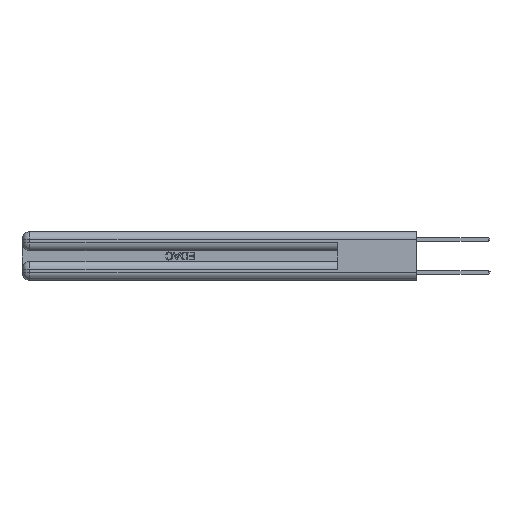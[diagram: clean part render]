
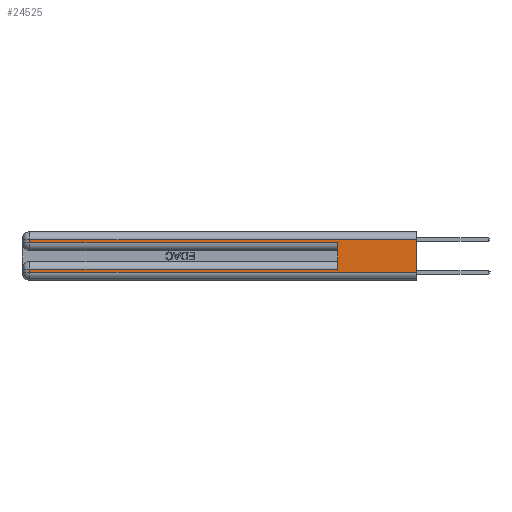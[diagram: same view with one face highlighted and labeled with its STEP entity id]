
A CAD part, left-side view. The second image highlights one B-rep face of the part: STEP entity #24525.
In plain terms, the highlighted planar face has unit normal (-1, 0, 0).
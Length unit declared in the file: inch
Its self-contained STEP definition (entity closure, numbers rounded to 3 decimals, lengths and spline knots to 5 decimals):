
#641 = CARTESIAN_POINT ( 'NONE',  ( 0., 0., 0.37 ) ) ;
#754 = DIRECTION ( 'NONE',  ( 0., 0., 1. ) ) ;
#1929 = CARTESIAN_POINT ( 'NONE',  ( 0., 2.94, 0.285 ) ) ;
#3793 = LINE ( 'NONE', #35618, #17306 ) ;
#3908 = DIRECTION ( 'NONE',  ( 0., 0., -1. ) ) ;
#4179 = EDGE_CURVE ( 'NONE', #4597, #15960, #12061, .T. ) ;
#4214 = CARTESIAN_POINT ( 'NONE',  ( 0., 0.6, 0.285 ) ) ;
#4295 = ORIENTED_EDGE ( 'NONE', *, *, #4179, .T. ) ;
#4597 = VERTEX_POINT ( 'NONE', #26328 ) ;
#4673 = EDGE_CURVE ( 'NONE', #29137, #15960, #22553, .T. ) ;
#4898 = VERTEX_POINT ( 'NONE', #36300 ) ;
#4946 = ORIENTED_EDGE ( 'NONE', *, *, #4673, .F. ) ;
#5827 = EDGE_CURVE ( 'NONE', #29381, #18650, #32218, .T. ) ;
#7454 = VECTOR ( 'NONE', #34073, 39.37008 ) ;
#7671 = ORIENTED_EDGE ( 'NONE', *, *, #17218, .T. ) ;
#8417 = ORIENTED_EDGE ( 'NONE', *, *, #13299, .T. ) ;
#9285 = DIRECTION ( 'NONE',  ( 0., 0., -1. ) ) ;
#10624 = DIRECTION ( 'NONE',  ( 0., 1., 0. ) ) ;
#10973 = LINE ( 'NONE', #28683, #23853 ) ;
#11108 = VECTOR ( 'NONE', #10624, 39.37008 ) ;
#11722 = LINE ( 'NONE', #12283, #33886 ) ;
#12061 = LINE ( 'NONE', #28634, #32073 ) ;
#12283 = CARTESIAN_POINT ( 'NONE',  ( 0., 0., 0.31 ) ) ;
#12311 = CARTESIAN_POINT ( 'NONE',  ( 0., 0., 0.31 ) ) ;
#13299 = EDGE_CURVE ( 'NONE', #29381, #4898, #33990, .T. ) ;
#15139 = VERTEX_POINT ( 'NONE', #24621 ) ;
#15486 = EDGE_CURVE ( 'NONE', #4898, #4597, #15737, .T. ) ;
#15737 = LINE ( 'NONE', #29707, #35317 ) ;
#15960 = VERTEX_POINT ( 'NONE', #30206 ) ;
#16243 = ORIENTED_EDGE ( 'NONE', *, *, #21794, .T. ) ;
#16978 = CARTESIAN_POINT ( 'NONE',  ( 0., 0.6, 0.085 ) ) ;
#17218 = EDGE_CURVE ( 'NONE', #28214, #18650, #10973, .T. ) ;
#17306 = VECTOR ( 'NONE', #24281, 39.37008 ) ;
#17945 = DIRECTION ( 'NONE',  ( 1., 0., 0. ) ) ;
#18056 = CARTESIAN_POINT ( 'NONE',  ( 0., 0.6, 0.145 ) ) ;
#18650 = VERTEX_POINT ( 'NONE', #4214 ) ;
#19034 = ORIENTED_EDGE ( 'NONE', *, *, #15486, .T. ) ;
#20773 = PLANE ( 'NONE',  #36339 ) ;
#21794 = EDGE_CURVE ( 'NONE', #29137, #15139, #11722, .T. ) ;
#22553 = LINE ( 'NONE', #28972, #7454 ) ;
#23207 = DIRECTION ( 'NONE',  ( 0., -1., 0. ) ) ;
#23533 = DIRECTION ( 'NONE',  ( 0., -1., 0. ) ) ;
#23766 = DIRECTION ( 'NONE',  ( 0., 1., 0. ) ) ;
#23853 = VECTOR ( 'NONE', #23207, 39.37008 ) ;
#24281 = DIRECTION ( 'NONE',  ( 0., 0., -1. ) ) ;
#24525 = ADVANCED_FACE ( 'NONE', ( #34930 ), #20773, .F. ) ;
#24563 = CARTESIAN_POINT ( 'NONE',  ( 0., 0., 0.085 ) ) ;
#24621 = CARTESIAN_POINT ( 'NONE',  ( 0., 2.94, 0.31 ) ) ;
#24792 = EDGE_LOOP ( 'NONE', ( #4946, #16243, #25158, #7671, #35066, #8417, #19034, #4295 ) ) ;
#25158 = ORIENTED_EDGE ( 'NONE', *, *, #31000, .T. ) ;
#25846 = VECTOR ( 'NONE', #754, 39.37008 ) ;
#26328 = CARTESIAN_POINT ( 'NONE',  ( 0., 2.94, 0.06 ) ) ;
#28214 = VERTEX_POINT ( 'NONE', #1929 ) ;
#28634 = CARTESIAN_POINT ( 'NONE',  ( 0., 0., 0.06 ) ) ;
#28683 = CARTESIAN_POINT ( 'NONE',  ( 0., 0., 0.285 ) ) ;
#28972 = CARTESIAN_POINT ( 'NONE',  ( 0., 0., 0.37 ) ) ;
#29137 = VERTEX_POINT ( 'NONE', #12311 ) ;
#29381 = VERTEX_POINT ( 'NONE', #16978 ) ;
#29707 = CARTESIAN_POINT ( 'NONE',  ( 0., 2.94, 0.37 ) ) ;
#30206 = CARTESIAN_POINT ( 'NONE',  ( 0., 0., 0.06 ) ) ;
#31000 = EDGE_CURVE ( 'NONE', #15139, #28214, #3793, .T. ) ;
#32073 = VECTOR ( 'NONE', #23533, 39.37008 ) ;
#32218 = LINE ( 'NONE', #18056, #25846 ) ;
#33886 = VECTOR ( 'NONE', #23766, 39.37008 ) ;
#33990 = LINE ( 'NONE', #24563, #11108 ) ;
#34073 = DIRECTION ( 'NONE',  ( 0., 0., -1. ) ) ;
#34930 = FACE_OUTER_BOUND ( 'NONE', #24792, .T. ) ;
#35066 = ORIENTED_EDGE ( 'NONE', *, *, #5827, .F. ) ;
#35317 = VECTOR ( 'NONE', #3908, 39.37008 ) ;
#35618 = CARTESIAN_POINT ( 'NONE',  ( 0., 2.94, 0.37 ) ) ;
#36300 = CARTESIAN_POINT ( 'NONE',  ( 0., 2.94, 0.085 ) ) ;
#36339 = AXIS2_PLACEMENT_3D ( 'NONE', #641, #17945, #9285 ) ;
